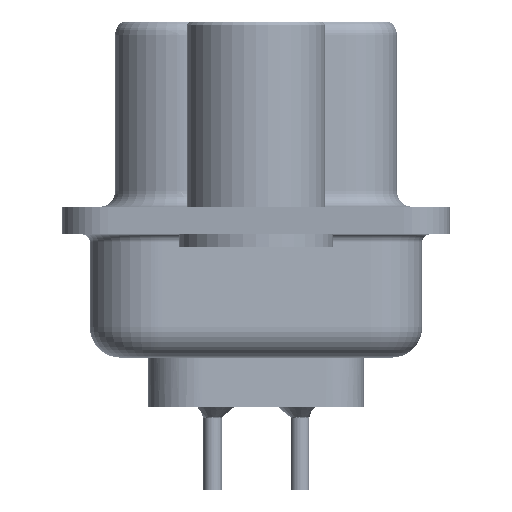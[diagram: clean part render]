
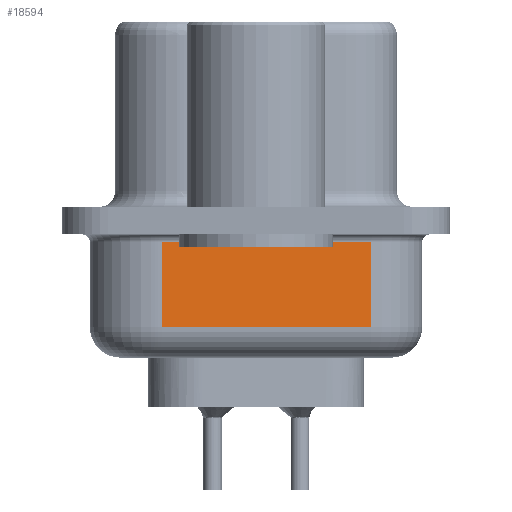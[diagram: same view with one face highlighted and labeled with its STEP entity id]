
A CAD part, left-side view. The second image highlights one B-rep face of the part: STEP entity #18594.
In plain terms, the highlighted planar face has unit normal (-0.985, -0.174, 0).
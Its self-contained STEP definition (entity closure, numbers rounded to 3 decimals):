
#2831 = VERTEX_POINT ( 'NONE', #14550 ) ;
#3339 = EDGE_CURVE ( 'NONE', #10930, #30185, #28857, .T. ) ;
#4292 = CARTESIAN_POINT ( 'NONE',  ( 2.88, 3.053, -3.45 ) ) ;
#4774 = DIRECTION ( 'NONE',  ( 0.174, -0.985, 0. ) ) ;
#4883 = EDGE_CURVE ( 'NONE', #9041, #10930, #24750, .T. ) ;
#6084 = VECTOR ( 'NONE', #4774, 1000. ) ;
#6890 = CARTESIAN_POINT ( 'NONE',  ( 2.88, 3.053, -4.45 ) ) ;
#8035 = CARTESIAN_POINT ( 'NONE',  ( 4.079, -3.747, -0.7 ) ) ;
#9041 = VERTEX_POINT ( 'NONE', #4292 ) ;
#9152 = PLANE ( 'NONE',  #29036 ) ;
#10930 = VERTEX_POINT ( 'NONE', #14016 ) ;
#10953 = VECTOR ( 'NONE', #11946, 1000. ) ;
#11609 = DIRECTION ( 'NONE',  ( 0.985, 0.174, 0. ) ) ;
#11840 = CARTESIAN_POINT ( 'NONE',  ( 4.079, -3.747, -4.45 ) ) ;
#11946 = DIRECTION ( 'NONE',  ( 0., 0., 1. ) ) ;
#12014 = EDGE_LOOP ( 'NONE', ( #22539, #28115, #13364, #21539 ) ) ;
#12341 = CARTESIAN_POINT ( 'NONE',  ( 2.88, 3.053, -0.7 ) ) ;
#12895 = EDGE_CURVE ( 'NONE', #30185, #2831, #18061, .T. ) ;
#13364 = ORIENTED_EDGE ( 'NONE', *, *, #3339, .T. ) ;
#13454 = FACE_OUTER_BOUND ( 'NONE', #12014, .T. ) ;
#14016 = CARTESIAN_POINT ( 'NONE',  ( 4.079, -3.747, -3.45 ) ) ;
#14550 = CARTESIAN_POINT ( 'NONE',  ( 2.88, 3.053, -0.7 ) ) ;
#15811 = LINE ( 'NONE', #19605, #27510 ) ;
#18061 = LINE ( 'NONE', #12341, #24990 ) ;
#18594 = ADVANCED_FACE ( 'NONE', ( #13454 ), #9152, .F. ) ;
#19605 = CARTESIAN_POINT ( 'NONE',  ( 2.88, 3.053, -4.45 ) ) ;
#21539 = ORIENTED_EDGE ( 'NONE', *, *, #12895, .T. ) ;
#22539 = ORIENTED_EDGE ( 'NONE', *, *, #23269, .F. ) ;
#23269 = EDGE_CURVE ( 'NONE', #9041, #2831, #15811, .T. ) ;
#23462 = CARTESIAN_POINT ( 'NONE',  ( 2.88, 3.053, -3.45 ) ) ;
#24750 = LINE ( 'NONE', #23462, #6084 ) ;
#24990 = VECTOR ( 'NONE', #26363, 1000. ) ;
#26363 = DIRECTION ( 'NONE',  ( -0.174, 0.985, 0. ) ) ;
#27510 = VECTOR ( 'NONE', #28993, 1000. ) ;
#27964 = DIRECTION ( 'NONE',  ( -0.174, 0.985, 0. ) ) ;
#28115 = ORIENTED_EDGE ( 'NONE', *, *, #4883, .T. ) ;
#28857 = LINE ( 'NONE', #11840, #10953 ) ;
#28993 = DIRECTION ( 'NONE',  ( 0., 0., 1. ) ) ;
#29036 = AXIS2_PLACEMENT_3D ( 'NONE', #6890, #11609, #27964 ) ;
#30185 = VERTEX_POINT ( 'NONE', #8035 ) ;
